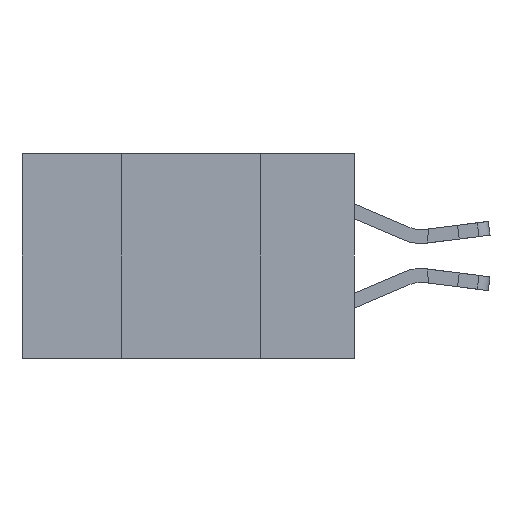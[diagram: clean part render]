
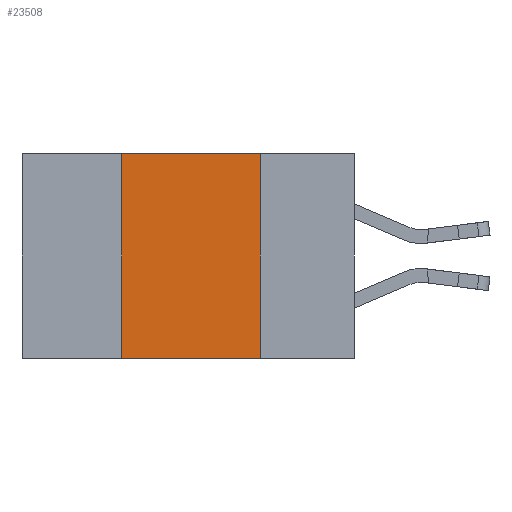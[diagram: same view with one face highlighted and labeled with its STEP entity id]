
A CAD part, left-side view. The second image highlights one B-rep face of the part: STEP entity #23508.
In plain terms, the highlighted planar face has unit normal (-1, 0, 0).
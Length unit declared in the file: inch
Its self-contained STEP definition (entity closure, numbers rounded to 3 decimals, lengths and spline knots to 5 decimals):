
#957 = DIRECTION ( 'NONE',  ( 1., 0., 0. ) ) ;
#971 = AXIS2_PLACEMENT_3D ( 'NONE', #4693, #957, #13972 ) ;
#1101 = EDGE_CURVE ( 'NONE', #21395, #10426, #10548, .T. ) ;
#2623 = VECTOR ( 'NONE', #23986, 39.37008 ) ;
#3752 = DIRECTION ( 'NONE',  ( 0., 0., 1. ) ) ;
#4693 = CARTESIAN_POINT ( 'NONE',  ( 0., 0.6, 0. ) ) ;
#5088 = CARTESIAN_POINT ( 'NONE',  ( 0., 0.17, 0. ) ) ;
#5672 = CARTESIAN_POINT ( 'NONE',  ( 0., 0.17, 0. ) ) ;
#5729 = VECTOR ( 'NONE', #19036, 39.37008 ) ;
#6664 = ORIENTED_EDGE ( 'NONE', *, *, #23816, .F. ) ;
#7316 = EDGE_CURVE ( 'NONE', #14273, #10426, #23273, .T. ) ;
#7491 = CARTESIAN_POINT ( 'NONE',  ( 0., 0.42, 0. ) ) ;
#8559 = DIRECTION ( 'NONE',  ( 0., -1., 0. ) ) ;
#9013 = CARTESIAN_POINT ( 'NONE',  ( 0., 0.6, -0.37 ) ) ;
#10426 = VERTEX_POINT ( 'NONE', #14694 ) ;
#10548 = LINE ( 'NONE', #5672, #5729 ) ;
#10643 = CARTESIAN_POINT ( 'NONE',  ( 0., 0.42, -0.37 ) ) ;
#12108 = PLANE ( 'NONE',  #971 ) ;
#13688 = EDGE_LOOP ( 'NONE', ( #14743, #16983, #6664, #15835 ) ) ;
#13796 = LINE ( 'NONE', #7491, #23575 ) ;
#13972 = DIRECTION ( 'NONE',  ( 0., 0., -1. ) ) ;
#14273 = VERTEX_POINT ( 'NONE', #10643 ) ;
#14694 = CARTESIAN_POINT ( 'NONE',  ( 0., 0.17, -0.37 ) ) ;
#14743 = ORIENTED_EDGE ( 'NONE', *, *, #1101, .F. ) ;
#15835 = ORIENTED_EDGE ( 'NONE', *, *, #7316, .T. ) ;
#16983 = ORIENTED_EDGE ( 'NONE', *, *, #19103, .F. ) ;
#18220 = VERTEX_POINT ( 'NONE', #21677 ) ;
#18998 = VECTOR ( 'NONE', #8559, 39.37008 ) ;
#19036 = DIRECTION ( 'NONE',  ( 0., 0., -1. ) ) ;
#19103 = EDGE_CURVE ( 'NONE', #18220, #21395, #22241, .T. ) ;
#20188 = FACE_OUTER_BOUND ( 'NONE', #13688, .T. ) ;
#21395 = VERTEX_POINT ( 'NONE', #5088 ) ;
#21677 = CARTESIAN_POINT ( 'NONE',  ( 0., 0.42, 0. ) ) ;
#22241 = LINE ( 'NONE', #23915, #2623 ) ;
#23273 = LINE ( 'NONE', #9013, #18998 ) ;
#23508 = ADVANCED_FACE ( 'NONE', ( #20188 ), #12108, .F. ) ;
#23575 = VECTOR ( 'NONE', #3752, 39.37008 ) ;
#23816 = EDGE_CURVE ( 'NONE', #14273, #18220, #13796, .T. ) ;
#23915 = CARTESIAN_POINT ( 'NONE',  ( 0., 0.6, 0. ) ) ;
#23986 = DIRECTION ( 'NONE',  ( 0., -1., 0. ) ) ;
